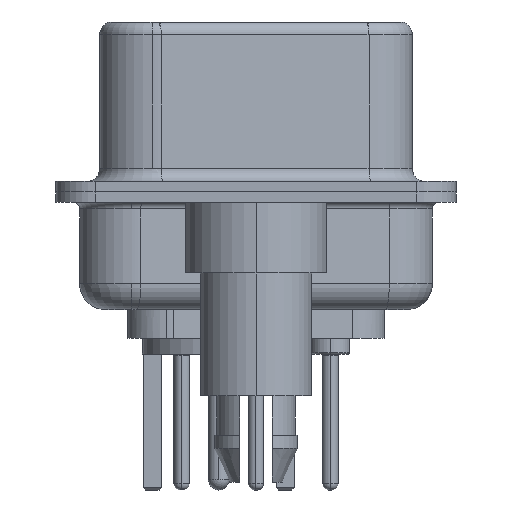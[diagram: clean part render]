
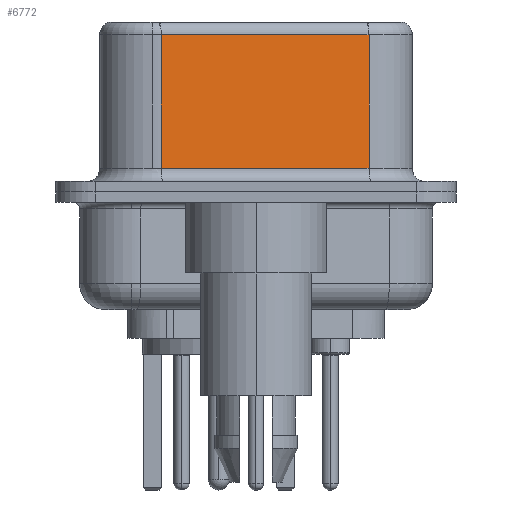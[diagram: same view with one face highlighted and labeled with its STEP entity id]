
A CAD part, left-side view. The second image highlights one B-rep face of the part: STEP entity #6772.
In plain terms, the highlighted planar face has unit normal (-0.985, -0.174, 0).
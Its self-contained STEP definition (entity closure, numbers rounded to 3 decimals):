
#497 = LINE ( 'NONE', #2343, #27595 ) ;
#1190 = VERTEX_POINT ( 'NONE', #19510 ) ;
#2343 = CARTESIAN_POINT ( 'NONE',  ( 5.132, -4.322, 6.52 ) ) ;
#2546 = ORIENTED_EDGE ( 'NONE', *, *, #12235, .T. ) ;
#2976 = CARTESIAN_POINT ( 'NONE',  ( 3.73, 3.628, 0.9 ) ) ;
#3154 = CARTESIAN_POINT ( 'NONE',  ( 5.132, -4.322, 6.02 ) ) ;
#6083 = EDGE_CURVE ( 'NONE', #17243, #11748, #497, .T. ) ;
#6568 = EDGE_CURVE ( 'NONE', #1190, #28757, #22209, .T. ) ;
#6772 = ADVANCED_FACE ( 'NONE', ( #10332 ), #10517, .F. ) ;
#7037 = CARTESIAN_POINT ( 'NONE',  ( 5.132, -4.322, 0.9 ) ) ;
#8298 = VECTOR ( 'NONE', #17590, 1000. ) ;
#10213 = DIRECTION ( 'NONE',  ( 0., 0., -1. ) ) ;
#10332 = FACE_OUTER_BOUND ( 'NONE', #21324, .T. ) ;
#10517 = PLANE ( 'NONE',  #12563 ) ;
#11748 = VERTEX_POINT ( 'NONE', #28261 ) ;
#11823 = LINE ( 'NONE', #30218, #31042 ) ;
#12235 = EDGE_CURVE ( 'NONE', #28757, #11748, #31110, .T. ) ;
#12391 = CARTESIAN_POINT ( 'NONE',  ( 3.73, 3.628, 6.52 ) ) ;
#12563 = AXIS2_PLACEMENT_3D ( 'NONE', #18261, #28836, #13185 ) ;
#13185 = DIRECTION ( 'NONE',  ( -0.174, 0.985, 0. ) ) ;
#17243 = VERTEX_POINT ( 'NONE', #3154 ) ;
#17590 = DIRECTION ( 'NONE',  ( 0., 0., -1. ) ) ;
#18261 = CARTESIAN_POINT ( 'NONE',  ( 5.132, -4.322, 6.52 ) ) ;
#19510 = CARTESIAN_POINT ( 'NONE',  ( 3.73, 3.628, 6.02 ) ) ;
#20947 = ORIENTED_EDGE ( 'NONE', *, *, #6083, .F. ) ;
#21324 = EDGE_LOOP ( 'NONE', ( #20947, #23691, #28841, #2546 ) ) ;
#22209 = LINE ( 'NONE', #12391, #8298 ) ;
#22715 = DIRECTION ( 'NONE',  ( 0.174, -0.985, 0. ) ) ;
#23366 = VECTOR ( 'NONE', #22715, 1000. ) ;
#23691 = ORIENTED_EDGE ( 'NONE', *, *, #32301, .T. ) ;
#27595 = VECTOR ( 'NONE', #10213, 1000. ) ;
#28261 = CARTESIAN_POINT ( 'NONE',  ( 5.132, -4.322, 0.9 ) ) ;
#28757 = VERTEX_POINT ( 'NONE', #2976 ) ;
#28836 = DIRECTION ( 'NONE',  ( 0.985, 0.174, 0. ) ) ;
#28841 = ORIENTED_EDGE ( 'NONE', *, *, #6568, .T. ) ;
#30218 = CARTESIAN_POINT ( 'NONE',  ( 5.132, -4.322, 6.02 ) ) ;
#31042 = VECTOR ( 'NONE', #32842, 1000. ) ;
#31110 = LINE ( 'NONE', #7037, #23366 ) ;
#32301 = EDGE_CURVE ( 'NONE', #17243, #1190, #11823, .T. ) ;
#32842 = DIRECTION ( 'NONE',  ( -0.174, 0.985, 0. ) ) ;
